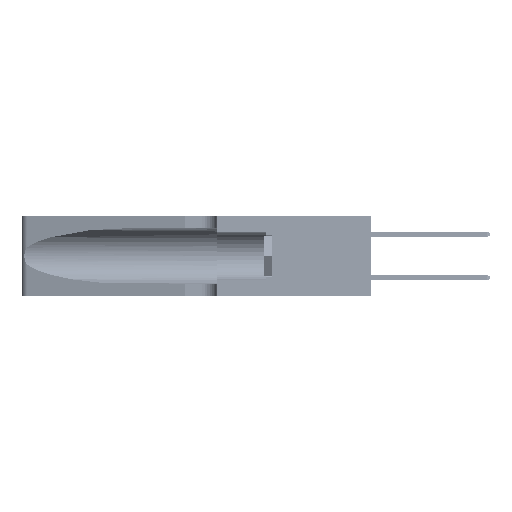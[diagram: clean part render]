
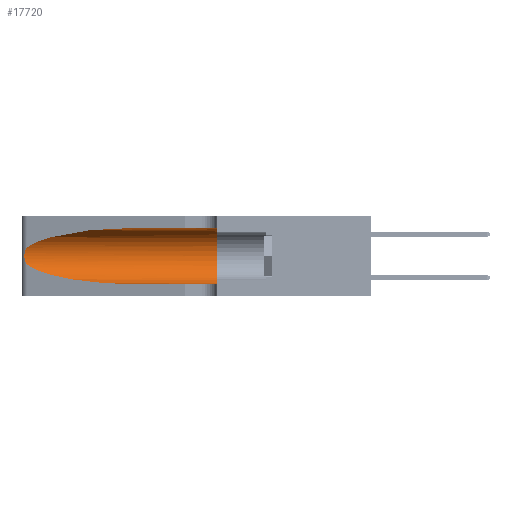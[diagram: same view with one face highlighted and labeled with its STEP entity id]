
A CAD part, left-side view. The second image highlights one B-rep face of the part: STEP entity #17720.
In plain terms, the highlighted cylindrical face has radius 3.308 mm (diameter 6.617 mm), a partial arc.
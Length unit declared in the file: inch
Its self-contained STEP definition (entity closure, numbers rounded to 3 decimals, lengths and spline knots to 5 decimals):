
#692 = CARTESIAN_POINT ( 'NONE',  ( 0.1305, 0.72297, 0.31525 ) ) ;
#1536 = EDGE_CURVE ( 'NONE', #35299, #52318, #17563, .T. ) ;
#2101 = CARTESIAN_POINT ( 'NONE',  ( 0.25555, 1.22993, 0.14849 ) ) ;
#2133 = B_SPLINE_CURVE_WITH_KNOTS ( 'NONE', 3,
 ( #27716, #44171, #48034, #52930, #52209, #2650, #52573, #27170, #39733, #31874, #6847, #39914, #2101, #11053 ),
 .UNSPECIFIED., .F., .F.,
 ( 4, 2, 2, 2, 2, 2, 4 ),
 ( 0., 0.00027, 0.00053, 0.00107, 0.0016, 0.00187, 0.00214 ),
 .UNSPECIFIED. ) ;
#2507 = CARTESIAN_POINT ( 'NONE',  ( 0.25487, 1.22718, 0.22369 ) ) ;
#2650 = CARTESIAN_POINT ( 'NONE',  ( 0.26018, 1.23835, 0.19895 ) ) ;
#2718 = FACE_OUTER_BOUND ( 'NONE', #32211, .T. ) ;
#6847 = CARTESIAN_POINT ( 'NONE',  ( 0.25789, 1.23486, 0.15765 ) ) ;
#7411 = EDGE_CURVE ( 'NONE', #40560, #7508, #35294, .T. ) ;
#7508 = VERTEX_POINT ( 'NONE', #51670 ) ;
#11053 = CARTESIAN_POINT ( 'NONE',  ( 0.25487, 1.22718, 0.14631 ) ) ;
#11991 = ORIENTED_EDGE ( 'NONE', *, *, #7411, .T. ) ;
#12564 = CARTESIAN_POINT ( 'NONE',  ( 0.18966, 0.96281, 0.05475 ) ) ;
#13067 = AXIS2_PLACEMENT_3D ( 'NONE', #30842, #22602, #35217 ) ;
#13796 = CARTESIAN_POINT ( 'NONE',  ( 0.2373, 1.15595, 0.28018 ) ) ;
#14014 = ORIENTED_EDGE ( 'NONE', *, *, #1536, .T. ) ;
#14154 = DIRECTION ( 'NONE',  ( 0., -1., 0. ) ) ;
#14476 = LINE ( 'NONE', #25637, #34080 ) ;
#16947 = CARTESIAN_POINT ( 'NONE',  ( 0.25487, 1.22718, 0.14631 ) ) ;
#17540 = ORIENTED_EDGE ( 'NONE', *, *, #40135, .T. ) ;
#17563 =( BOUNDED_CURVE ( )  B_SPLINE_CURVE ( 3, ( #26222, #26962, #13796, #51639 ),
 .UNSPECIFIED., .F., .T. ) 
 B_SPLINE_CURVE_WITH_KNOTS ( ( 4, 4 ),
 ( 1.5708, 2.84003 ),
 .UNSPECIFIED. ) 
 CURVE ( )  GEOMETRIC_REPRESENTATION_ITEM ( )  RATIONAL_B_SPLINE_CURVE ( ( 1., 0.87, 0.87, 1. ) ) 
 REPRESENTATION_ITEM ( '' )  );
#17720 = ADVANCED_FACE ( 'NONE', ( #2718 ), #34753, .F. ) ;
#19138 = ORIENTED_EDGE ( 'NONE', *, *, #35511, .F. ) ;
#21506 = CARTESIAN_POINT ( 'NONE',  ( 0.2373, 1.15595, 0.08982 ) ) ;
#22305 = ORIENTED_EDGE ( 'NONE', *, *, #42397, .T. ) ;
#22602 = DIRECTION ( 'NONE',  ( 0., 1., 0. ) ) ;
#24555 = DIRECTION ( 'NONE',  ( 0., -1., 0. ) ) ;
#25637 = CARTESIAN_POINT ( 'NONE',  ( 0.1305, 1.61858, 0.05475 ) ) ;
#26222 = CARTESIAN_POINT ( 'NONE',  ( 0.1305, 0.72297, 0.31525 ) ) ;
#26962 = CARTESIAN_POINT ( 'NONE',  ( 0.18966, 0.96281, 0.31525 ) ) ;
#27170 = CARTESIAN_POINT ( 'NONE',  ( 0.26075, 1.23896, 0.178 ) ) ;
#27716 = CARTESIAN_POINT ( 'NONE',  ( 0.25487, 1.22718, 0.22369 ) ) ;
#30588 = DIRECTION ( 'NONE',  ( 0., 0., -1. ) ) ;
#30842 = CARTESIAN_POINT ( 'NONE',  ( 0.1305, 0.35, 0.185 ) ) ;
#31874 = CARTESIAN_POINT ( 'NONE',  ( 0.25856, 1.23593, 0.16098 ) ) ;
#32211 = EDGE_LOOP ( 'NONE', ( #14014, #17540, #11991, #22305, #19138, #38226 ) ) ;
#32447 = LINE ( 'NONE', #49470, #45595 ) ;
#34080 = VECTOR ( 'NONE', #37881, 39.37008 ) ;
#34753 = CYLINDRICAL_SURFACE ( 'NONE', #40266, 0.13025 ) ;
#34786 = CARTESIAN_POINT ( 'NONE',  ( 0.25487, 1.22718, 0.14631 ) ) ;
#35217 = DIRECTION ( 'NONE',  ( 0., 0., 1. ) ) ;
#35294 =( BOUNDED_CURVE ( )  B_SPLINE_CURVE ( 3, ( #16947, #21506, #12564, #50777 ),
 .UNSPECIFIED., .F., .F. ) 
 B_SPLINE_CURVE_WITH_KNOTS ( ( 4, 4 ),
 ( 3.44316, 4.71239 ),
 .UNSPECIFIED. ) 
 CURVE ( )  GEOMETRIC_REPRESENTATION_ITEM ( )  RATIONAL_B_SPLINE_CURVE ( ( 1., 0.87, 0.87, 1. ) ) 
 REPRESENTATION_ITEM ( '' )  );
#35299 = VERTEX_POINT ( 'NONE', #692 ) ;
#35511 = EDGE_CURVE ( 'NONE', #49662, #50026, #42320, .T. ) ;
#37881 = DIRECTION ( 'NONE',  ( 0., -1., 0. ) ) ;
#38226 = ORIENTED_EDGE ( 'NONE', *, *, #52673, .F. ) ;
#39733 = CARTESIAN_POINT ( 'NONE',  ( 0.26017, 1.23833, 0.17102 ) ) ;
#39914 = CARTESIAN_POINT ( 'NONE',  ( 0.25639, 1.23186, 0.15144 ) ) ;
#40135 = EDGE_CURVE ( 'NONE', #52318, #40560, #2133, .T. ) ;
#40266 = AXIS2_PLACEMENT_3D ( 'NONE', #51641, #14154, #30588 ) ;
#40560 = VERTEX_POINT ( 'NONE', #34786 ) ;
#42320 = CIRCLE ( 'NONE', #13067, 0.13025 ) ;
#42397 = EDGE_CURVE ( 'NONE', #7508, #50026, #14476, .T. ) ;
#44171 = CARTESIAN_POINT ( 'NONE',  ( 0.25555, 1.22994, 0.2215 ) ) ;
#45595 = VECTOR ( 'NONE', #24555, 39.37008 ) ;
#48034 = CARTESIAN_POINT ( 'NONE',  ( 0.25639, 1.23184, 0.21858 ) ) ;
#49470 = CARTESIAN_POINT ( 'NONE',  ( 0.1305, 1.61858, 0.31525 ) ) ;
#49662 = VERTEX_POINT ( 'NONE', #51993 ) ;
#50026 = VERTEX_POINT ( 'NONE', #53964 ) ;
#50777 = CARTESIAN_POINT ( 'NONE',  ( 0.1305, 0.72297, 0.05475 ) ) ;
#51639 = CARTESIAN_POINT ( 'NONE',  ( 0.25487, 1.22718, 0.22369 ) ) ;
#51641 = CARTESIAN_POINT ( 'NONE',  ( 0.1305, 1.61858, 0.185 ) ) ;
#51670 = CARTESIAN_POINT ( 'NONE',  ( 0.1305, 0.72297, 0.05475 ) ) ;
#51993 = CARTESIAN_POINT ( 'NONE',  ( 0.1305, 0.35, 0.31525 ) ) ;
#52209 = CARTESIAN_POINT ( 'NONE',  ( 0.25854, 1.2359, 0.20912 ) ) ;
#52318 = VERTEX_POINT ( 'NONE', #2507 ) ;
#52573 = CARTESIAN_POINT ( 'NONE',  ( 0.26075, 1.23896, 0.19203 ) ) ;
#52673 = EDGE_CURVE ( 'NONE', #35299, #49662, #32447, .T. ) ;
#52930 = CARTESIAN_POINT ( 'NONE',  ( 0.25787, 1.23484, 0.2124 ) ) ;
#53964 = CARTESIAN_POINT ( 'NONE',  ( 0.1305, 0.35, 0.05475 ) ) ;
